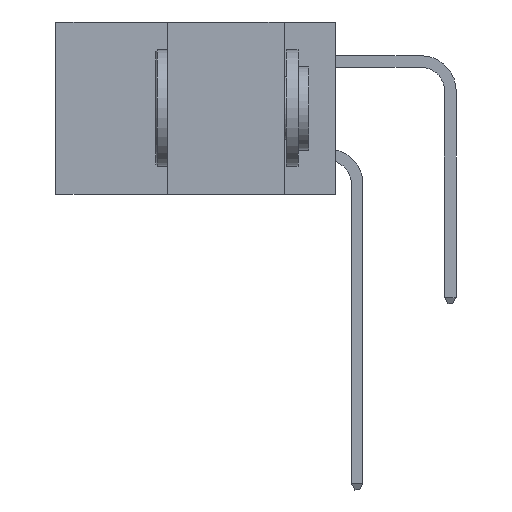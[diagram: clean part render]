
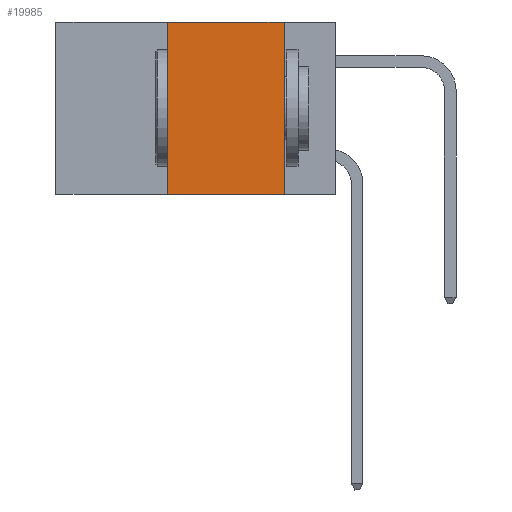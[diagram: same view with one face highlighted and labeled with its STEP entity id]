
A CAD part, left-side view. The second image highlights one B-rep face of the part: STEP entity #19985.
In plain terms, the highlighted planar face has unit normal (-1, 0, 0).
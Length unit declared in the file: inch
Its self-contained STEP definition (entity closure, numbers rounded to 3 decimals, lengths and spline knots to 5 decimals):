
#65 = AXIS2_PLACEMENT_3D ( 'NONE', #14387, #3421, #16203 ) ;
#143 = VECTOR ( 'NONE', #9617, 39.37008 ) ;
#949 = EDGE_CURVE ( 'NONE', #19976, #16669, #20112, .T. ) ;
#1068 = ORIENTED_EDGE ( 'NONE', *, *, #8268, .F. ) ;
#1088 = ORIENTED_EDGE ( 'NONE', *, *, #949, .F. ) ;
#1494 = PLANE ( 'NONE',  #65 ) ;
#1575 = VECTOR ( 'NONE', #9211, 39.37008 ) ;
#1623 = ORIENTED_EDGE ( 'NONE', *, *, #12918, .T. ) ;
#3421 = DIRECTION ( 'NONE',  ( 1., 0., 0. ) ) ;
#3813 = DIRECTION ( 'NONE',  ( 0., -1., 0. ) ) ;
#4503 = VERTEX_POINT ( 'NONE', #21701 ) ;
#5175 = CARTESIAN_POINT ( 'NONE',  ( 0., 0.11, 0. ) ) ;
#5975 = CARTESIAN_POINT ( 'NONE',  ( 0., 0.11, -0.37 ) ) ;
#8268 = EDGE_CURVE ( 'NONE', #16998, #19976, #8638, .T. ) ;
#8638 = LINE ( 'NONE', #16600, #18843 ) ;
#8789 = CARTESIAN_POINT ( 'NONE',  ( 0., 0.36, 0. ) ) ;
#9211 = DIRECTION ( 'NONE',  ( 0., -1., 0. ) ) ;
#9617 = DIRECTION ( 'NONE',  ( 0., 0., 1. ) ) ;
#10673 = LINE ( 'NONE', #22285, #143 ) ;
#11113 = VECTOR ( 'NONE', #23469, 39.37008 ) ;
#11571 = EDGE_CURVE ( 'NONE', #4503, #16998, #10673, .T. ) ;
#12918 = EDGE_CURVE ( 'NONE', #4503, #16669, #16245, .T. ) ;
#14387 = CARTESIAN_POINT ( 'NONE',  ( 0., 0.6, 0. ) ) ;
#15557 = FACE_OUTER_BOUND ( 'NONE', #22566, .T. ) ;
#16203 = DIRECTION ( 'NONE',  ( 0., 0., -1. ) ) ;
#16245 = LINE ( 'NONE', #20012, #1575 ) ;
#16600 = CARTESIAN_POINT ( 'NONE',  ( 0., 0.6, 0. ) ) ;
#16669 = VERTEX_POINT ( 'NONE', #5975 ) ;
#16998 = VERTEX_POINT ( 'NONE', #8789 ) ;
#18843 = VECTOR ( 'NONE', #3813, 39.37008 ) ;
#19976 = VERTEX_POINT ( 'NONE', #5175 ) ;
#19985 = ADVANCED_FACE ( 'NONE', ( #15557 ), #1494, .F. ) ;
#20012 = CARTESIAN_POINT ( 'NONE',  ( 0., 0.6, -0.37 ) ) ;
#20112 = LINE ( 'NONE', #23306, #11113 ) ;
#21603 = ORIENTED_EDGE ( 'NONE', *, *, #11571, .F. ) ;
#21701 = CARTESIAN_POINT ( 'NONE',  ( 0., 0.36, -0.37 ) ) ;
#22285 = CARTESIAN_POINT ( 'NONE',  ( 0., 0.36, 0. ) ) ;
#22566 = EDGE_LOOP ( 'NONE', ( #1088, #1068, #21603, #1623 ) ) ;
#23306 = CARTESIAN_POINT ( 'NONE',  ( 0., 0.11, 0. ) ) ;
#23469 = DIRECTION ( 'NONE',  ( 0., 0., -1. ) ) ;
